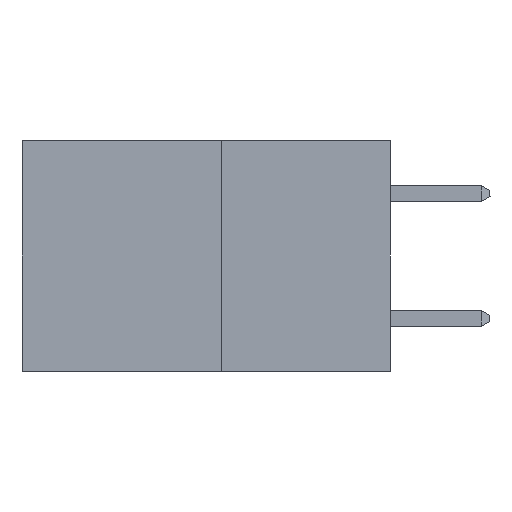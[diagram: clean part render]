
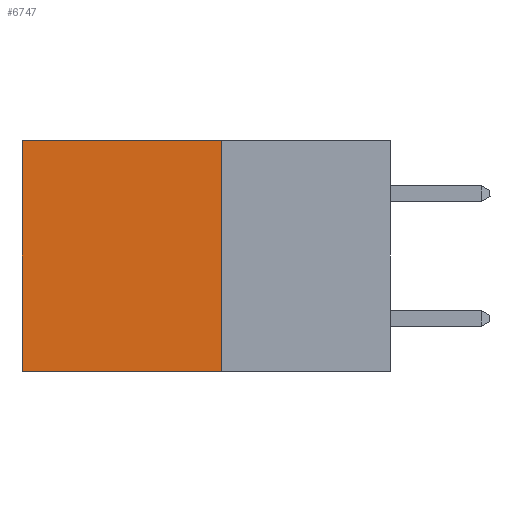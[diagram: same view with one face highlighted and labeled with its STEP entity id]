
A CAD part, left-side view. The second image highlights one B-rep face of the part: STEP entity #6747.
In plain terms, the highlighted planar face has unit normal (-1, 0, 0).
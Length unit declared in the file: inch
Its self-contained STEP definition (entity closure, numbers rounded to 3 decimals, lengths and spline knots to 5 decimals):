
#228 = LINE ( 'NONE', #16946, #10893 ) ;
#814 = VERTEX_POINT ( 'NONE', #8123 ) ;
#911 = VERTEX_POINT ( 'NONE', #6228 ) ;
#1660 = LINE ( 'NONE', #15010, #8643 ) ;
#2173 = CARTESIAN_POINT ( 'NONE',  ( 0.277, 0.27, -0.37 ) ) ;
#2282 = CARTESIAN_POINT ( 'NONE',  ( 0.277, 0.27, 0. ) ) ;
#3483 = CARTESIAN_POINT ( 'NONE',  ( 0.277, 0.27, -0.37 ) ) ;
#4373 = EDGE_CURVE ( 'NONE', #814, #17540, #1660, .T. ) ;
#4817 = AXIS2_PLACEMENT_3D ( 'NONE', #2173, #12109, #11745 ) ;
#5096 = DIRECTION ( 'NONE',  ( 0., 0., -1. ) ) ;
#5266 = EDGE_LOOP ( 'NONE', ( #17007, #15150, #8077, #17055 ) ) ;
#5769 = EDGE_CURVE ( 'NONE', #12773, #911, #15870, .T. ) ;
#6228 = CARTESIAN_POINT ( 'NONE',  ( 0.277, 0.27, -0.37 ) ) ;
#6747 = ADVANCED_FACE ( 'NONE', ( #7633 ), #12174, .F. ) ;
#7086 = CARTESIAN_POINT ( 'NONE',  ( 0.277, 0.27, -0.37 ) ) ;
#7219 = DIRECTION ( 'NONE',  ( 0., 0., -1. ) ) ;
#7633 = FACE_OUTER_BOUND ( 'NONE', #5266, .T. ) ;
#7695 = DIRECTION ( 'NONE',  ( 0., 1., 0. ) ) ;
#8077 = ORIENTED_EDGE ( 'NONE', *, *, #5769, .F. ) ;
#8123 = CARTESIAN_POINT ( 'NONE',  ( 0.277, 0.59, 0. ) ) ;
#8643 = VECTOR ( 'NONE', #7219, 39.37008 ) ;
#10550 = LINE ( 'NONE', #3483, #14205 ) ;
#10585 = EDGE_CURVE ( 'NONE', #12773, #814, #228, .T. ) ;
#10893 = VECTOR ( 'NONE', #12861, 39.37008 ) ;
#11745 = DIRECTION ( 'NONE',  ( 0., 0., -1. ) ) ;
#12109 = DIRECTION ( 'NONE',  ( 1., 0., 0. ) ) ;
#12174 = PLANE ( 'NONE',  #4817 ) ;
#12773 = VERTEX_POINT ( 'NONE', #2282 ) ;
#12861 = DIRECTION ( 'NONE',  ( 0., 1., 0. ) ) ;
#13955 = EDGE_CURVE ( 'NONE', #911, #17540, #10550, .T. ) ;
#14205 = VECTOR ( 'NONE', #7695, 39.37008 ) ;
#15010 = CARTESIAN_POINT ( 'NONE',  ( 0.277, 0.59, -0.37 ) ) ;
#15150 = ORIENTED_EDGE ( 'NONE', *, *, #13955, .F. ) ;
#15455 = VECTOR ( 'NONE', #5096, 39.37008 ) ;
#15870 = LINE ( 'NONE', #7086, #15455 ) ;
#16615 = CARTESIAN_POINT ( 'NONE',  ( 0.277, 0.59, -0.37 ) ) ;
#16946 = CARTESIAN_POINT ( 'NONE',  ( 0.277, 0.27, 0. ) ) ;
#17007 = ORIENTED_EDGE ( 'NONE', *, *, #4373, .T. ) ;
#17055 = ORIENTED_EDGE ( 'NONE', *, *, #10585, .T. ) ;
#17540 = VERTEX_POINT ( 'NONE', #16615 ) ;
